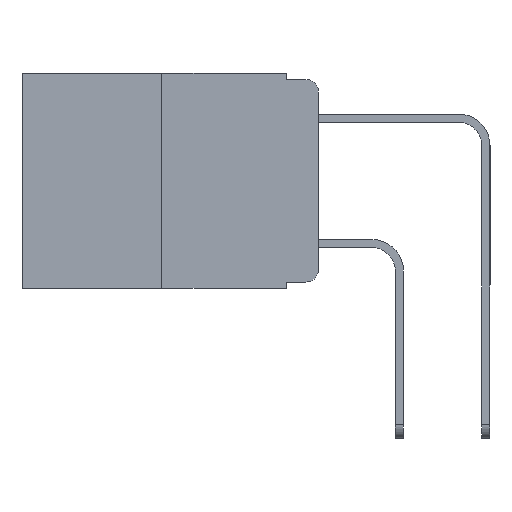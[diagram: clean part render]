
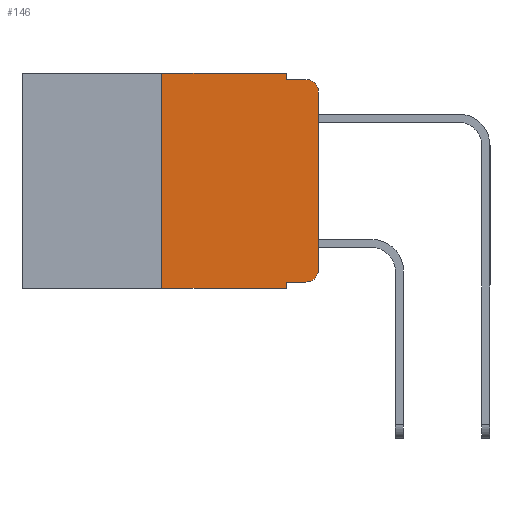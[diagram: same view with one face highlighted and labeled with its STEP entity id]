
A CAD part, left-side view. The second image highlights one B-rep face of the part: STEP entity #146.
In plain terms, the highlighted planar face has unit normal (-1, 0, 0).
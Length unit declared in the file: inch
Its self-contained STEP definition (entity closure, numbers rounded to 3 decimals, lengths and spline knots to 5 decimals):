
#146 = ADVANCED_FACE ( 'NONE', ( #6340 ), #1960, .F. ) ;
#153 = LINE ( 'NONE', #11105, #7199 ) ;
#233 = VECTOR ( 'NONE', #10199, 39.37008 ) ;
#244 = VERTEX_POINT ( 'NONE', #15939 ) ;
#461 = EDGE_CURVE ( 'NONE', #6852, #8557, #10202, .T. ) ;
#921 = VERTEX_POINT ( 'NONE', #7745 ) ;
#945 = CIRCLE ( 'NONE', #12407, 0.02 ) ;
#1097 = ORIENTED_EDGE ( 'NONE', *, *, #7951, .F. ) ;
#1291 = CARTESIAN_POINT ( 'NONE',  ( 0., 0.25, -0.343 ) ) ;
#1670 = DIRECTION ( 'NONE',  ( 0., 0., -1. ) ) ;
#1954 = ORIENTED_EDGE ( 'NONE', *, *, #6902, .F. ) ;
#1960 = PLANE ( 'NONE',  #7602 ) ;
#2234 = VERTEX_POINT ( 'NONE', #12467 ) ;
#2574 = EDGE_CURVE ( 'NONE', #15713, #9099, #4054, .T. ) ;
#2673 = CARTESIAN_POINT ( 'NONE',  ( 0., 0.051, -0.343 ) ) ;
#2837 = DIRECTION ( 'NONE',  ( 0., -1., 0. ) ) ;
#3124 = CIRCLE ( 'NONE', #7860, 0.02 ) ;
#3319 = ORIENTED_EDGE ( 'NONE', *, *, #15367, .F. ) ;
#3438 = ORIENTED_EDGE ( 'NONE', *, *, #2574, .T. ) ;
#3452 = LINE ( 'NONE', #3746, #6740 ) ;
#3510 = ORIENTED_EDGE ( 'NONE', *, *, #13609, .T. ) ;
#3746 = CARTESIAN_POINT ( 'NONE',  ( 0., 0.051, -0.333 ) ) ;
#3897 = CARTESIAN_POINT ( 'NONE',  ( 0., 0.473, 0. ) ) ;
#4017 = EDGE_CURVE ( 'NONE', #9099, #921, #945, .T. ) ;
#4054 = LINE ( 'NONE', #11095, #233 ) ;
#4444 = DIRECTION ( 'NONE',  ( -1., 0., 0. ) ) ;
#4458 = DIRECTION ( 'NONE',  ( 0., 0., 1. ) ) ;
#5034 = DIRECTION ( 'NONE',  ( 0., 0., -1. ) ) ;
#5100 = CARTESIAN_POINT ( 'NONE',  ( 0., 0.25, 0. ) ) ;
#5151 = DIRECTION ( 'NONE',  ( 0., -1., 0. ) ) ;
#5335 = DIRECTION ( 'NONE',  ( -1., 0., 0. ) ) ;
#5391 = ORIENTED_EDGE ( 'NONE', *, *, #10822, .T. ) ;
#5457 = DIRECTION ( 'NONE',  ( 0., 0., -1. ) ) ;
#5771 = ORIENTED_EDGE ( 'NONE', *, *, #15540, .F. ) ;
#5864 = VECTOR ( 'NONE', #7061, 39.37008 ) ;
#5957 = ORIENTED_EDGE ( 'NONE', *, *, #8683, .T. ) ;
#6340 = FACE_OUTER_BOUND ( 'NONE', #11360, .T. ) ;
#6702 = CARTESIAN_POINT ( 'NONE',  ( 0., 0.02, -0.03 ) ) ;
#6740 = VECTOR ( 'NONE', #5151, 39.37008 ) ;
#6793 = VECTOR ( 'NONE', #16710, 39.37008 ) ;
#6852 = VERTEX_POINT ( 'NONE', #14142 ) ;
#6902 = EDGE_CURVE ( 'NONE', #10798, #9424, #13506, .T. ) ;
#7033 = VERTEX_POINT ( 'NONE', #1291 ) ;
#7061 = DIRECTION ( 'NONE',  ( 0., -1., 0. ) ) ;
#7199 = VECTOR ( 'NONE', #1670, 39.37008 ) ;
#7208 = CARTESIAN_POINT ( 'NONE',  ( 0., 0.25, 0. ) ) ;
#7602 = AXIS2_PLACEMENT_3D ( 'NONE', #8453, #11018, #5034 ) ;
#7745 = CARTESIAN_POINT ( 'NONE',  ( 0., 0.02, -0.01 ) ) ;
#7860 = AXIS2_PLACEMENT_3D ( 'NONE', #12220, #4444, #13479 ) ;
#7951 = EDGE_CURVE ( 'NONE', #7033, #10798, #11333, .T. ) ;
#8443 = DIRECTION ( 'NONE',  ( 0., 0., -1. ) ) ;
#8453 = CARTESIAN_POINT ( 'NONE',  ( 0., 0.473, 0. ) ) ;
#8557 = VERTEX_POINT ( 'NONE', #2673 ) ;
#8612 = CARTESIAN_POINT ( 'NONE',  ( 0., 0.051, 0. ) ) ;
#8683 = EDGE_CURVE ( 'NONE', #7033, #8557, #9352, .T. ) ;
#9099 = VERTEX_POINT ( 'NONE', #9193 ) ;
#9193 = CARTESIAN_POINT ( 'NONE',  ( 0., 0., -0.03 ) ) ;
#9352 = LINE ( 'NONE', #12105, #5864 ) ;
#9379 = ORIENTED_EDGE ( 'NONE', *, *, #4017, .T. ) ;
#9424 = VERTEX_POINT ( 'NONE', #9652 ) ;
#9619 = LINE ( 'NONE', #15884, #13309 ) ;
#9652 = CARTESIAN_POINT ( 'NONE',  ( 0., 0.051, 0. ) ) ;
#10199 = DIRECTION ( 'NONE',  ( 0., 0., 1. ) ) ;
#10202 = LINE ( 'NONE', #8612, #13866 ) ;
#10798 = VERTEX_POINT ( 'NONE', #5100 ) ;
#10822 = EDGE_CURVE ( 'NONE', #6852, #2234, #3452, .T. ) ;
#10955 = VECTOR ( 'NONE', #4458, 39.37008 ) ;
#11018 = DIRECTION ( 'NONE',  ( 1., 0., 0. ) ) ;
#11095 = CARTESIAN_POINT ( 'NONE',  ( 0., 0., 0. ) ) ;
#11105 = CARTESIAN_POINT ( 'NONE',  ( 0., 0.051, 0. ) ) ;
#11332 = ORIENTED_EDGE ( 'NONE', *, *, #461, .F. ) ;
#11333 = LINE ( 'NONE', #7208, #10955 ) ;
#11360 = EDGE_LOOP ( 'NONE', ( #3438, #9379, #3319, #5771, #1954, #1097, #5957, #11332, #5391, #3510 ) ) ;
#12105 = CARTESIAN_POINT ( 'NONE',  ( 0., 0.473, -0.343 ) ) ;
#12220 = CARTESIAN_POINT ( 'NONE',  ( 0., 0.02, -0.313 ) ) ;
#12407 = AXIS2_PLACEMENT_3D ( 'NONE', #6702, #5335, #5457 ) ;
#12467 = CARTESIAN_POINT ( 'NONE',  ( 0., 0.02, -0.333 ) ) ;
#13309 = VECTOR ( 'NONE', #2837, 39.37008 ) ;
#13479 = DIRECTION ( 'NONE',  ( 0., 0., -1. ) ) ;
#13506 = LINE ( 'NONE', #3897, #6793 ) ;
#13609 = EDGE_CURVE ( 'NONE', #2234, #15713, #3124, .T. ) ;
#13866 = VECTOR ( 'NONE', #8443, 39.37008 ) ;
#14142 = CARTESIAN_POINT ( 'NONE',  ( 0., 0.051, -0.333 ) ) ;
#15216 = CARTESIAN_POINT ( 'NONE',  ( 0., 0., -0.313 ) ) ;
#15367 = EDGE_CURVE ( 'NONE', #244, #921, #9619, .T. ) ;
#15540 = EDGE_CURVE ( 'NONE', #9424, #244, #153, .T. ) ;
#15713 = VERTEX_POINT ( 'NONE', #15216 ) ;
#15884 = CARTESIAN_POINT ( 'NONE',  ( 0., 0.051, -0.01 ) ) ;
#15939 = CARTESIAN_POINT ( 'NONE',  ( 0., 0.051, -0.01 ) ) ;
#16710 = DIRECTION ( 'NONE',  ( 0., -1., 0. ) ) ;
